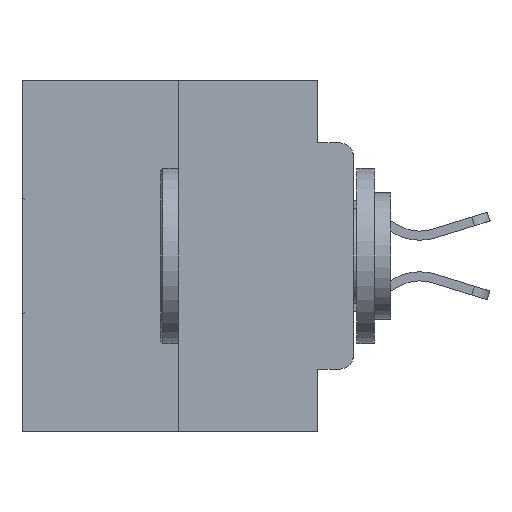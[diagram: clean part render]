
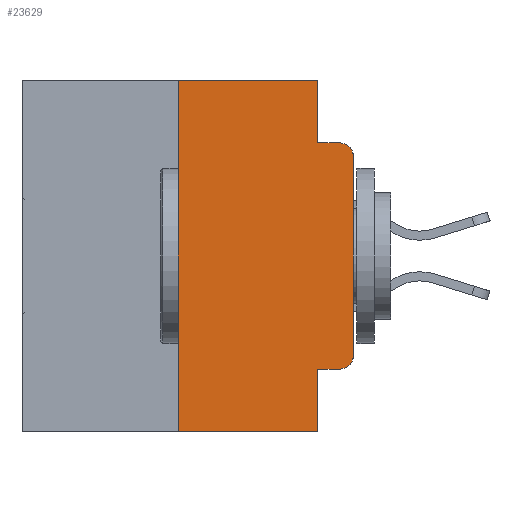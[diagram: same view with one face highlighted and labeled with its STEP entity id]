
A CAD part, left-side view. The second image highlights one B-rep face of the part: STEP entity #23629.
In plain terms, the highlighted planar face has unit normal (-1, 0, 0).
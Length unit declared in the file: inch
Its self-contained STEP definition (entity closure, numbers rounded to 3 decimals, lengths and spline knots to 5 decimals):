
#170 = VECTOR ( 'NONE', #21303, 39.37008 ) ;
#240 = ORIENTED_EDGE ( 'NONE', *, *, #10127, .T. ) ;
#300 = VECTOR ( 'NONE', #5251, 39.37008 ) ;
#470 = AXIS2_PLACEMENT_3D ( 'NONE', #19347, #5373, #21704 ) ;
#863 = DIRECTION ( 'NONE',  ( 0., 0., 1. ) ) ;
#873 = DIRECTION ( 'NONE',  ( -1., 0., 0. ) ) ;
#2005 = EDGE_CURVE ( 'NONE', #2102, #6402, #19666, .T. ) ;
#2102 = VERTEX_POINT ( 'NONE', #6018 ) ;
#2499 = CARTESIAN_POINT ( 'NONE',  ( 0., 0., 0. ) ) ;
#2564 = CARTESIAN_POINT ( 'NONE',  ( 0., 0.02, -0.0885 ) ) ;
#3576 = VERTEX_POINT ( 'NONE', #2564 ) ;
#3633 = EDGE_CURVE ( 'NONE', #27338, #28587, #6088, .T. ) ;
#4041 = EDGE_CURVE ( 'NONE', #2102, #10941, #20314, .T. ) ;
#4264 = CARTESIAN_POINT ( 'NONE',  ( 0., 0.051, 0. ) ) ;
#4530 = ORIENTED_EDGE ( 'NONE', *, *, #26165, .T. ) ;
#5251 = DIRECTION ( 'NONE',  ( 0., 0., -1. ) ) ;
#5278 = EDGE_CURVE ( 'NONE', #28587, #3576, #11584, .T. ) ;
#5373 = DIRECTION ( 'NONE',  ( 1., 0., 0. ) ) ;
#5627 = CARTESIAN_POINT ( 'NONE',  ( 0., 0.051, 0. ) ) ;
#6018 = CARTESIAN_POINT ( 'NONE',  ( 0., 0.25, -0.5 ) ) ;
#6038 = ORIENTED_EDGE ( 'NONE', *, *, #11638, .T. ) ;
#6088 = LINE ( 'NONE', #5627, #300 ) ;
#6112 = EDGE_CURVE ( 'NONE', #6402, #27338, #14939, .T. ) ;
#6212 = CARTESIAN_POINT ( 'NONE',  ( 0., 0.25, 0. ) ) ;
#6241 = CIRCLE ( 'NONE', #12100, 0.02 ) ;
#6402 = VERTEX_POINT ( 'NONE', #6212 ) ;
#6813 = LINE ( 'NONE', #8086, #25334 ) ;
#7316 = DIRECTION ( 'NONE',  ( 0., -1., 0. ) ) ;
#8086 = CARTESIAN_POINT ( 'NONE',  ( 0., 0.051, 0. ) ) ;
#8145 = CARTESIAN_POINT ( 'NONE',  ( 0., 0., -0.3915 ) ) ;
#9058 = ORIENTED_EDGE ( 'NONE', *, *, #3633, .F. ) ;
#9242 = CARTESIAN_POINT ( 'NONE',  ( 0., 0.051, -0.5 ) ) ;
#9286 = CARTESIAN_POINT ( 'NONE',  ( 0., 0.473, 0. ) ) ;
#9948 = CIRCLE ( 'NONE', #10093, 0.02 ) ;
#10093 = AXIS2_PLACEMENT_3D ( 'NONE', #25158, #11311, #27488 ) ;
#10127 = EDGE_CURVE ( 'NONE', #27393, #3576, #6241, .T. ) ;
#10321 = CARTESIAN_POINT ( 'NONE',  ( 0., 0.02, -0.4115 ) ) ;
#10941 = VERTEX_POINT ( 'NONE', #9242 ) ;
#11025 = CARTESIAN_POINT ( 'NONE',  ( 0., 0.473, -0.5 ) ) ;
#11209 = CARTESIAN_POINT ( 'NONE',  ( 0., 0.051, -0.0885 ) ) ;
#11311 = DIRECTION ( 'NONE',  ( -1., 0., 0. ) ) ;
#11584 = LINE ( 'NONE', #12972, #17706 ) ;
#11601 = DIRECTION ( 'NONE',  ( 0., -1., 0. ) ) ;
#11621 = VECTOR ( 'NONE', #7316, 39.37008 ) ;
#11638 = EDGE_CURVE ( 'NONE', #11828, #27393, #19095, .T. ) ;
#11828 = VERTEX_POINT ( 'NONE', #8145 ) ;
#12100 = AXIS2_PLACEMENT_3D ( 'NONE', #15130, #873, #17457 ) ;
#12849 = CARTESIAN_POINT ( 'NONE',  ( 0., 0.25, 0. ) ) ;
#12972 = CARTESIAN_POINT ( 'NONE',  ( 0., 0.051, -0.0885 ) ) ;
#13551 = VECTOR ( 'NONE', #863, 39.37008 ) ;
#13889 = CARTESIAN_POINT ( 'NONE',  ( 0., 0., -0.1085 ) ) ;
#14219 = VECTOR ( 'NONE', #11601, 39.37008 ) ;
#14913 = VECTOR ( 'NONE', #27208, 39.37008 ) ;
#14939 = LINE ( 'NONE', #9286, #14219 ) ;
#15130 = CARTESIAN_POINT ( 'NONE',  ( 0., 0.02, -0.1085 ) ) ;
#17457 = DIRECTION ( 'NONE',  ( 0., 0., -1. ) ) ;
#17706 = VECTOR ( 'NONE', #26831, 39.37008 ) ;
#19095 = LINE ( 'NONE', #2499, #170 ) ;
#19153 = ORIENTED_EDGE ( 'NONE', *, *, #5278, .F. ) ;
#19347 = CARTESIAN_POINT ( 'NONE',  ( 0., 0.473, 0. ) ) ;
#19602 = DIRECTION ( 'NONE',  ( 0., 0., -1. ) ) ;
#19666 = LINE ( 'NONE', #12849, #13551 ) ;
#19959 = VERTEX_POINT ( 'NONE', #10321 ) ;
#20252 = ORIENTED_EDGE ( 'NONE', *, *, #4041, .T. ) ;
#20314 = LINE ( 'NONE', #11025, #14913 ) ;
#21303 = DIRECTION ( 'NONE',  ( 0., 0., 1. ) ) ;
#21345 = ORIENTED_EDGE ( 'NONE', *, *, #6112, .F. ) ;
#21704 = DIRECTION ( 'NONE',  ( 0., 0., -1. ) ) ;
#22992 = FACE_OUTER_BOUND ( 'NONE', #26751, .T. ) ;
#23190 = ORIENTED_EDGE ( 'NONE', *, *, #24643, .T. ) ;
#23554 = ORIENTED_EDGE ( 'NONE', *, *, #2005, .F. ) ;
#23569 = CARTESIAN_POINT ( 'NONE',  ( 0., 0.051, -0.4115 ) ) ;
#23629 = ADVANCED_FACE ( 'NONE', ( #22992 ), #23953, .F. ) ;
#23948 = LINE ( 'NONE', #23569, #11621 ) ;
#23953 = PLANE ( 'NONE',  #470 ) ;
#24643 = EDGE_CURVE ( 'NONE', #19959, #11828, #9948, .T. ) ;
#25158 = CARTESIAN_POINT ( 'NONE',  ( 0., 0.02, -0.3915 ) ) ;
#25334 = VECTOR ( 'NONE', #19602, 39.37008 ) ;
#26165 = EDGE_CURVE ( 'NONE', #28092, #19959, #23948, .T. ) ;
#26439 = ORIENTED_EDGE ( 'NONE', *, *, #27719, .F. ) ;
#26751 = EDGE_LOOP ( 'NONE', ( #6038, #240, #19153, #9058, #21345, #23554, #20252, #26439, #4530, #23190 ) ) ;
#26831 = DIRECTION ( 'NONE',  ( 0., -1., 0. ) ) ;
#27208 = DIRECTION ( 'NONE',  ( 0., -1., 0. ) ) ;
#27338 = VERTEX_POINT ( 'NONE', #4264 ) ;
#27393 = VERTEX_POINT ( 'NONE', #13889 ) ;
#27488 = DIRECTION ( 'NONE',  ( 0., 0., -1. ) ) ;
#27719 = EDGE_CURVE ( 'NONE', #28092, #10941, #6813, .T. ) ;
#28092 = VERTEX_POINT ( 'NONE', #30196 ) ;
#28587 = VERTEX_POINT ( 'NONE', #11209 ) ;
#30196 = CARTESIAN_POINT ( 'NONE',  ( 0., 0.051, -0.4115 ) ) ;
